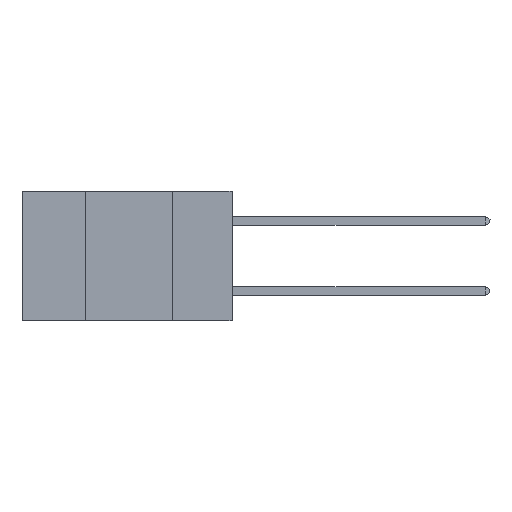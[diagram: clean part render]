
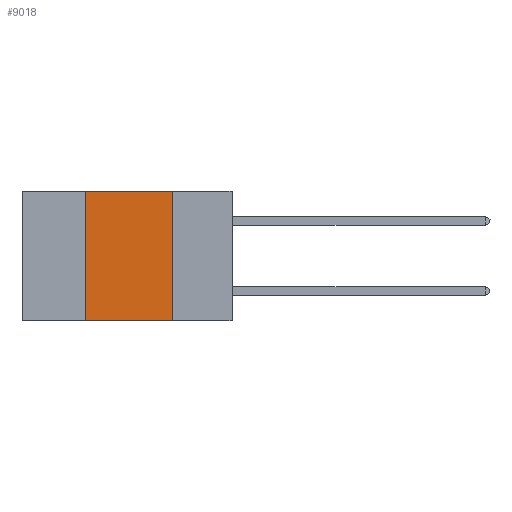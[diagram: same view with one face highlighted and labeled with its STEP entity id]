
A CAD part, left-side view. The second image highlights one B-rep face of the part: STEP entity #9018.
In plain terms, the highlighted planar face has unit normal (-1, 0, 0).
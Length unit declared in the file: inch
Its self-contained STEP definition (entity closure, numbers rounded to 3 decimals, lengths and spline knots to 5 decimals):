
#14 = VECTOR ( 'NONE', #6912, 39.37008 ) ;
#365 = ORIENTED_EDGE ( 'NONE', *, *, #473, .T. ) ;
#473 = EDGE_CURVE ( 'NONE', #3219, #10470, #8365, .T. ) ;
#977 = EDGE_CURVE ( 'NONE', #6525, #10470, #5826, .T. ) ;
#1487 = LINE ( 'NONE', #6243, #5194 ) ;
#2622 = CARTESIAN_POINT ( 'NONE',  ( 0., 0.6, -0.37 ) ) ;
#3219 = VERTEX_POINT ( 'NONE', #8979 ) ;
#3466 = ORIENTED_EDGE ( 'NONE', *, *, #12345, .F. ) ;
#3504 = CARTESIAN_POINT ( 'NONE',  ( 0., 0.17, -0.37 ) ) ;
#4378 = EDGE_CURVE ( 'NONE', #3219, #12120, #7915, .T. ) ;
#5191 = PLANE ( 'NONE',  #9951 ) ;
#5194 = VECTOR ( 'NONE', #9209, 39.37008 ) ;
#5398 = VECTOR ( 'NONE', #6708, 39.37008 ) ;
#5826 = LINE ( 'NONE', #7789, #5398 ) ;
#6243 = CARTESIAN_POINT ( 'NONE',  ( 0., 0.6, 0. ) ) ;
#6525 = VERTEX_POINT ( 'NONE', #11494 ) ;
#6708 = DIRECTION ( 'NONE',  ( 0., 0., -1. ) ) ;
#6912 = DIRECTION ( 'NONE',  ( 0., 0., 1. ) ) ;
#6919 = FACE_OUTER_BOUND ( 'NONE', #10529, .T. ) ;
#6982 = DIRECTION ( 'NONE',  ( 0., 0., -1. ) ) ;
#7789 = CARTESIAN_POINT ( 'NONE',  ( 0., 0.17, 0. ) ) ;
#7915 = LINE ( 'NONE', #11842, #14 ) ;
#7975 = DIRECTION ( 'NONE',  ( 1., 0., 0. ) ) ;
#8365 = LINE ( 'NONE', #2622, #9824 ) ;
#8493 = DIRECTION ( 'NONE',  ( 0., -1., 0. ) ) ;
#8914 = ORIENTED_EDGE ( 'NONE', *, *, #977, .F. ) ;
#8979 = CARTESIAN_POINT ( 'NONE',  ( 0., 0.42, -0.37 ) ) ;
#9018 = ADVANCED_FACE ( 'NONE', ( #6919 ), #5191, .F. ) ;
#9209 = DIRECTION ( 'NONE',  ( 0., -1., 0. ) ) ;
#9824 = VECTOR ( 'NONE', #8493, 39.37008 ) ;
#9951 = AXIS2_PLACEMENT_3D ( 'NONE', #11032, #7975, #6982 ) ;
#10470 = VERTEX_POINT ( 'NONE', #3504 ) ;
#10529 = EDGE_LOOP ( 'NONE', ( #8914, #3466, #10783, #365 ) ) ;
#10783 = ORIENTED_EDGE ( 'NONE', *, *, #4378, .F. ) ;
#11032 = CARTESIAN_POINT ( 'NONE',  ( 0., 0.6, 0. ) ) ;
#11494 = CARTESIAN_POINT ( 'NONE',  ( 0., 0.17, 0. ) ) ;
#11842 = CARTESIAN_POINT ( 'NONE',  ( 0., 0.42, 0. ) ) ;
#11938 = CARTESIAN_POINT ( 'NONE',  ( 0., 0.42, 0. ) ) ;
#12120 = VERTEX_POINT ( 'NONE', #11938 ) ;
#12345 = EDGE_CURVE ( 'NONE', #12120, #6525, #1487, .T. ) ;
